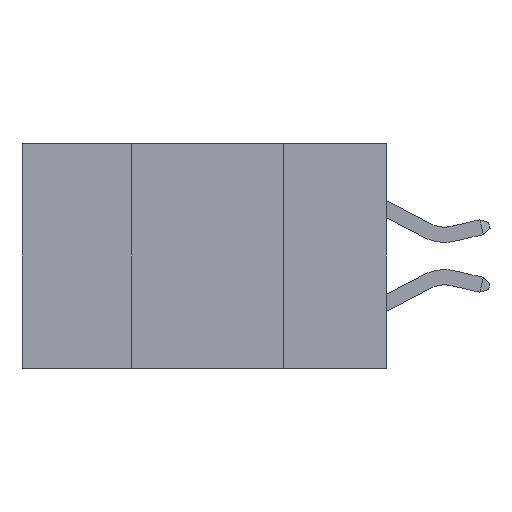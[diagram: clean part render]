
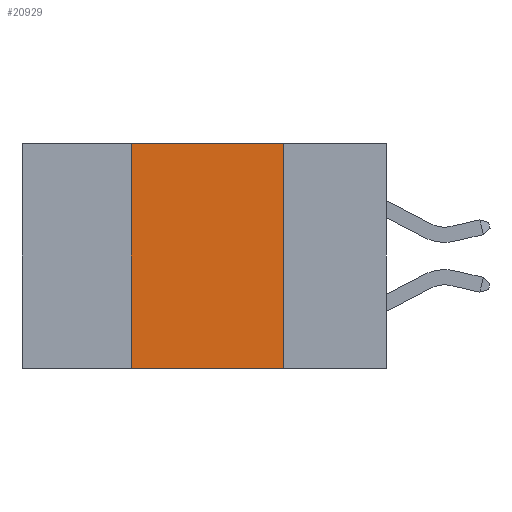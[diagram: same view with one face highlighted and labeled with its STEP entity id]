
A CAD part, left-side view. The second image highlights one B-rep face of the part: STEP entity #20929.
In plain terms, the highlighted planar face has unit normal (-1, 0, 0).
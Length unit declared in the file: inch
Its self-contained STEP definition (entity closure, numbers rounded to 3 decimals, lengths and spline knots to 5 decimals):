
#27 = DIRECTION ( 'NONE',  ( 0., 0., 1. ) ) ;
#1270 = VECTOR ( 'NONE', #3016, 39.37008 ) ;
#1844 = VECTOR ( 'NONE', #27, 39.37008 ) ;
#1847 = ORIENTED_EDGE ( 'NONE', *, *, #11446, .F. ) ;
#1855 = VERTEX_POINT ( 'NONE', #19135 ) ;
#3016 = DIRECTION ( 'NONE',  ( 0., -1., 0. ) ) ;
#3141 = CARTESIAN_POINT ( 'NONE',  ( 0., 0.42, 0. ) ) ;
#4601 = CARTESIAN_POINT ( 'NONE',  ( 0., 0.6, 0. ) ) ;
#4956 = VECTOR ( 'NONE', #22408, 39.37008 ) ;
#6229 = LINE ( 'NONE', #12619, #1844 ) ;
#6478 = DIRECTION ( 'NONE',  ( 1., 0., 0. ) ) ;
#6794 = ORIENTED_EDGE ( 'NONE', *, *, #10302, .F. ) ;
#7490 = VERTEX_POINT ( 'NONE', #19477 ) ;
#7886 = VERTEX_POINT ( 'NONE', #3141 ) ;
#7911 = EDGE_LOOP ( 'NONE', ( #6794, #1847, #19967, #19447 ) ) ;
#8696 = CARTESIAN_POINT ( 'NONE',  ( 0., 0.17, -0.37 ) ) ;
#10302 = EDGE_CURVE ( 'NONE', #11191, #7490, #19362, .T. ) ;
#11191 = VERTEX_POINT ( 'NONE', #13239 ) ;
#11446 = EDGE_CURVE ( 'NONE', #7886, #11191, #18250, .T. ) ;
#11540 = FACE_OUTER_BOUND ( 'NONE', #7911, .T. ) ;
#12115 = DIRECTION ( 'NONE',  ( 0., -1., 0. ) ) ;
#12619 = CARTESIAN_POINT ( 'NONE',  ( 0., 0.42, -0.37 ) ) ;
#13239 = CARTESIAN_POINT ( 'NONE',  ( 0., 0.17, 0. ) ) ;
#13623 = CARTESIAN_POINT ( 'NONE',  ( 0., 0.6, -0.37 ) ) ;
#14884 = EDGE_CURVE ( 'NONE', #1855, #7886, #6229, .T. ) ;
#15079 = PLANE ( 'NONE',  #21035 ) ;
#16074 = EDGE_CURVE ( 'NONE', #1855, #7490, #19464, .T. ) ;
#18250 = LINE ( 'NONE', #22367, #22225 ) ;
#18538 = DIRECTION ( 'NONE',  ( 0., 0., -1. ) ) ;
#19135 = CARTESIAN_POINT ( 'NONE',  ( 0., 0.42, -0.37 ) ) ;
#19362 = LINE ( 'NONE', #8696, #4956 ) ;
#19447 = ORIENTED_EDGE ( 'NONE', *, *, #16074, .T. ) ;
#19464 = LINE ( 'NONE', #13623, #1270 ) ;
#19477 = CARTESIAN_POINT ( 'NONE',  ( 0., 0.17, -0.37 ) ) ;
#19967 = ORIENTED_EDGE ( 'NONE', *, *, #14884, .F. ) ;
#20929 = ADVANCED_FACE ( 'NONE', ( #11540 ), #15079, .F. ) ;
#21035 = AXIS2_PLACEMENT_3D ( 'NONE', #4601, #6478, #18538 ) ;
#22225 = VECTOR ( 'NONE', #12115, 39.37008 ) ;
#22367 = CARTESIAN_POINT ( 'NONE',  ( 0., 0.6, 0. ) ) ;
#22408 = DIRECTION ( 'NONE',  ( 0., 0., -1. ) ) ;
